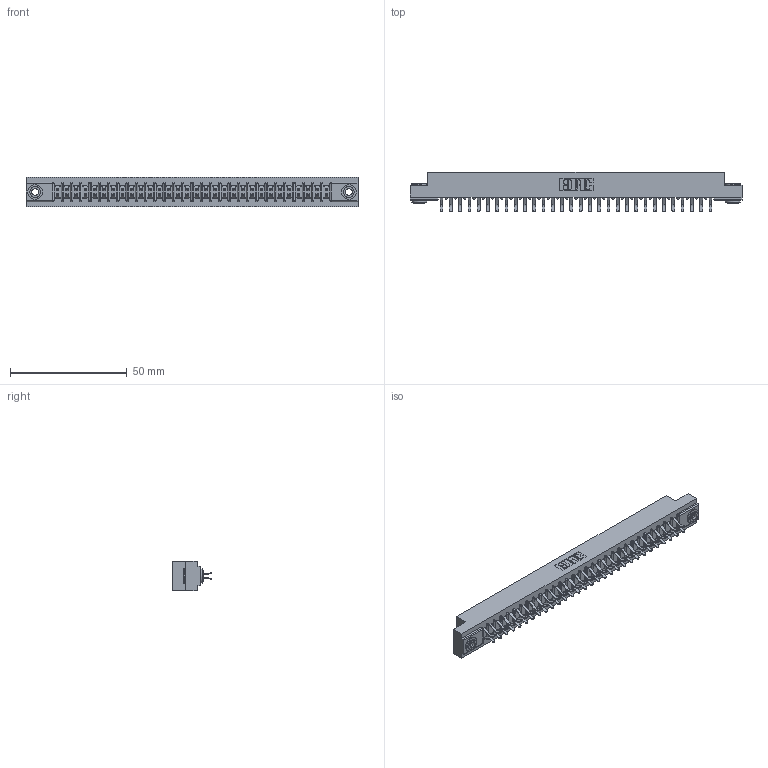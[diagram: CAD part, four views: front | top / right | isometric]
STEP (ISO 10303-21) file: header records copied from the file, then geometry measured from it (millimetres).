
FILE_DESCRIPTION (( 'STEP AP203' ), '1' );
FILE_NAME ('357-060-556-203.STEP', '2018-08-12T15:06:11', ( '' ), ( '' ), 'SwSTEP 2.0', 'SolidWorks 2016', '' );
FILE_SCHEMA (( 'CONFIG_CONTROL_DESIGN' ));
Length unit declared in the file: inch
Products named in the file (4): 307 Part_.156 Dia Mounting Holes; 307-290-001_556; 345-250-002_345-250-002-102; 357-060-556-203
Assembly tree (63 placements, depth 2):
  357-060-556-203
    307 Part_.156 Dia Mounting Holes
    307-290-001_556  x60
    345-250-002_345-250-002-102  x2
Bounding box: 141.88 x 16.97 x 12.7 mm (x, y, z)
Volume: 14993.1 mm3; surface area: 18195.2 mm2
Topology: 63 solids, 63 shells, 3201 faces, 8955 edges, 5802 vertices
Faces by surface type: plane 2074, cylinder 1057, sphere 62, cone 8
Entity records: 29327 total; most frequent: CARTESIAN_POINT 4783, ORIENTED_EDGE 4730, DIRECTION 4705, EDGE_CURVE 2365, VECTOR 1801, LINE 1801, VERTEX_POINT 1530, AXIS2_PLACEMENT_3D 1452
